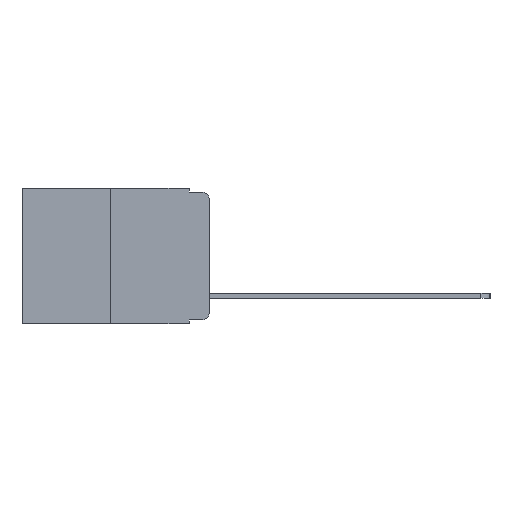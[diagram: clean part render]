
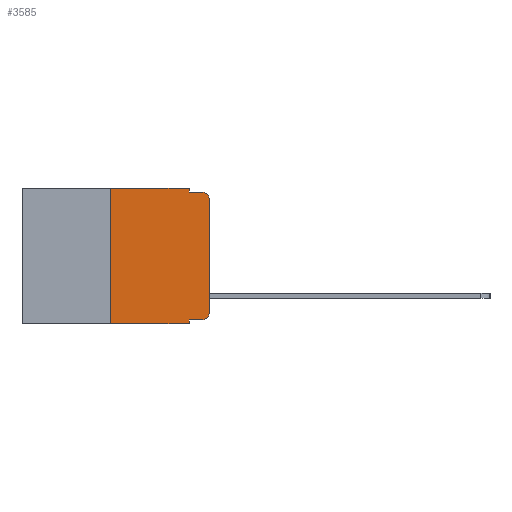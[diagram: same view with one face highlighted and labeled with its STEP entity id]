
A CAD part, left-side view. The second image highlights one B-rep face of the part: STEP entity #3585.
In plain terms, the highlighted planar face has unit normal (-1, 0, 0).
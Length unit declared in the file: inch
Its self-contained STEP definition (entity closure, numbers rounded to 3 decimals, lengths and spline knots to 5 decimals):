
#495 = LINE ( 'NONE', #16200, #16521 ) ;
#686 = EDGE_CURVE ( 'NONE', #1658, #749, #4327, .T. ) ;
#749 = VERTEX_POINT ( 'NONE', #12650 ) ;
#1012 = EDGE_CURVE ( 'NONE', #11154, #9003, #2589, .T. ) ;
#1107 = AXIS2_PLACEMENT_3D ( 'NONE', #9656, #19105, #10004 ) ;
#1211 = DIRECTION ( 'NONE',  ( 0., 0., -1. ) ) ;
#1265 = EDGE_CURVE ( 'NONE', #7196, #11154, #18304, .T. ) ;
#1481 = EDGE_CURVE ( 'NONE', #6351, #13529, #6319, .T. ) ;
#1658 = VERTEX_POINT ( 'NONE', #12062 ) ;
#2589 = LINE ( 'NONE', #7166, #6343 ) ;
#2643 = CARTESIAN_POINT ( 'NONE',  ( 0., 0.051, -0.01 ) ) ;
#3567 = CARTESIAN_POINT ( 'NONE',  ( 0., 0.051, 0. ) ) ;
#3585 = ADVANCED_FACE ( 'NONE', ( #17737 ), #5269, .F. ) ;
#3880 = CARTESIAN_POINT ( 'NONE',  ( 0., 0.051, 0. ) ) ;
#4211 = EDGE_CURVE ( 'NONE', #15313, #1658, #12962, .T. ) ;
#4293 = DIRECTION ( 'NONE',  ( 0., -1., 0. ) ) ;
#4327 = LINE ( 'NONE', #2643, #8088 ) ;
#4381 = AXIS2_PLACEMENT_3D ( 'NONE', #16010, #6828, #17540 ) ;
#5174 = VECTOR ( 'NONE', #9913, 39.37008 ) ;
#5269 = PLANE ( 'NONE',  #1107 ) ;
#5274 = EDGE_CURVE ( 'NONE', #10589, #7196, #19846, .T. ) ;
#5311 = ORIENTED_EDGE ( 'NONE', *, *, #9049, .T. ) ;
#6238 = EDGE_CURVE ( 'NONE', #10589, #17149, #10287, .T. ) ;
#6319 = LINE ( 'NONE', #12327, #14492 ) ;
#6343 = VECTOR ( 'NONE', #11746, 39.37008 ) ;
#6351 = VERTEX_POINT ( 'NONE', #18071 ) ;
#6630 = VECTOR ( 'NONE', #14754, 39.37008 ) ;
#6666 = VECTOR ( 'NONE', #15663, 39.37008 ) ;
#6828 = DIRECTION ( 'NONE',  ( -1., 0., 0. ) ) ;
#6833 = EDGE_CURVE ( 'NONE', #13529, #15313, #495, .T. ) ;
#7166 = CARTESIAN_POINT ( 'NONE',  ( 0., 0., 0. ) ) ;
#7196 = VERTEX_POINT ( 'NONE', #7988 ) ;
#7717 = ORIENTED_EDGE ( 'NONE', *, *, #1481, .F. ) ;
#7988 = CARTESIAN_POINT ( 'NONE',  ( 0., 0.02, -0.333 ) ) ;
#8055 = CARTESIAN_POINT ( 'NONE',  ( 0., 0.051, -0.333 ) ) ;
#8088 = VECTOR ( 'NONE', #4293, 39.37008 ) ;
#8312 = LINE ( 'NONE', #16942, #15941 ) ;
#9003 = VERTEX_POINT ( 'NONE', #19855 ) ;
#9049 = EDGE_CURVE ( 'NONE', #6351, #17149, #8312, .T. ) ;
#9237 = ORIENTED_EDGE ( 'NONE', *, *, #12660, .T. ) ;
#9313 = CARTESIAN_POINT ( 'NONE',  ( 0., 0.051, 0. ) ) ;
#9331 = ORIENTED_EDGE ( 'NONE', *, *, #4211, .F. ) ;
#9450 = DIRECTION ( 'NONE',  ( 0., 0., 1. ) ) ;
#9603 = ORIENTED_EDGE ( 'NONE', *, *, #6238, .F. ) ;
#9656 = CARTESIAN_POINT ( 'NONE',  ( 0., 0.473, 0. ) ) ;
#9775 = ORIENTED_EDGE ( 'NONE', *, *, #1012, .T. ) ;
#9913 = DIRECTION ( 'NONE',  ( 0., 0., -1. ) ) ;
#10004 = DIRECTION ( 'NONE',  ( 0., 0., -1. ) ) ;
#10287 = LINE ( 'NONE', #3880, #6630 ) ;
#10589 = VERTEX_POINT ( 'NONE', #11546 ) ;
#10629 = DIRECTION ( 'NONE',  ( -1., 0., 0. ) ) ;
#11154 = VERTEX_POINT ( 'NONE', #16678 ) ;
#11158 = AXIS2_PLACEMENT_3D ( 'NONE', #19736, #10629, #1211 ) ;
#11170 = ORIENTED_EDGE ( 'NONE', *, *, #1265, .T. ) ;
#11546 = CARTESIAN_POINT ( 'NONE',  ( 0., 0.051, -0.333 ) ) ;
#11746 = DIRECTION ( 'NONE',  ( 0., 0., 1. ) ) ;
#12062 = CARTESIAN_POINT ( 'NONE',  ( 0., 0.051, -0.01 ) ) ;
#12327 = CARTESIAN_POINT ( 'NONE',  ( 0., 0.25, 0. ) ) ;
#12650 = CARTESIAN_POINT ( 'NONE',  ( 0., 0.02, -0.01 ) ) ;
#12660 = EDGE_CURVE ( 'NONE', #9003, #749, #15117, .T. ) ;
#12962 = LINE ( 'NONE', #3567, #5174 ) ;
#13529 = VERTEX_POINT ( 'NONE', #16658 ) ;
#14492 = VECTOR ( 'NONE', #9450, 39.37008 ) ;
#14754 = DIRECTION ( 'NONE',  ( 0., 0., -1. ) ) ;
#15117 = CIRCLE ( 'NONE', #4381, 0.02 ) ;
#15313 = VERTEX_POINT ( 'NONE', #9313 ) ;
#15663 = DIRECTION ( 'NONE',  ( 0., -1., 0. ) ) ;
#15941 = VECTOR ( 'NONE', #18456, 39.37008 ) ;
#16010 = CARTESIAN_POINT ( 'NONE',  ( 0., 0.02, -0.03 ) ) ;
#16148 = ORIENTED_EDGE ( 'NONE', *, *, #5274, .T. ) ;
#16200 = CARTESIAN_POINT ( 'NONE',  ( 0., 0.473, 0. ) ) ;
#16265 = DIRECTION ( 'NONE',  ( 0., -1., 0. ) ) ;
#16521 = VECTOR ( 'NONE', #16265, 39.37008 ) ;
#16658 = CARTESIAN_POINT ( 'NONE',  ( 0., 0.25, 0. ) ) ;
#16678 = CARTESIAN_POINT ( 'NONE',  ( 0., 0., -0.313 ) ) ;
#16942 = CARTESIAN_POINT ( 'NONE',  ( 0., 0.473, -0.343 ) ) ;
#17149 = VERTEX_POINT ( 'NONE', #18220 ) ;
#17540 = DIRECTION ( 'NONE',  ( 0., 0., -1. ) ) ;
#17606 = ORIENTED_EDGE ( 'NONE', *, *, #6833, .F. ) ;
#17737 = FACE_OUTER_BOUND ( 'NONE', #18385, .T. ) ;
#18071 = CARTESIAN_POINT ( 'NONE',  ( 0., 0.25, -0.343 ) ) ;
#18220 = CARTESIAN_POINT ( 'NONE',  ( 0., 0.051, -0.343 ) ) ;
#18304 = CIRCLE ( 'NONE', #11158, 0.02 ) ;
#18385 = EDGE_LOOP ( 'NONE', ( #9775, #9237, #19295, #9331, #17606, #7717, #5311, #9603, #16148, #11170 ) ) ;
#18456 = DIRECTION ( 'NONE',  ( 0., -1., 0. ) ) ;
#19105 = DIRECTION ( 'NONE',  ( 1., 0., 0. ) ) ;
#19295 = ORIENTED_EDGE ( 'NONE', *, *, #686, .F. ) ;
#19736 = CARTESIAN_POINT ( 'NONE',  ( 0., 0.02, -0.313 ) ) ;
#19846 = LINE ( 'NONE', #8055, #6666 ) ;
#19855 = CARTESIAN_POINT ( 'NONE',  ( 0., 0., -0.03 ) ) ;
